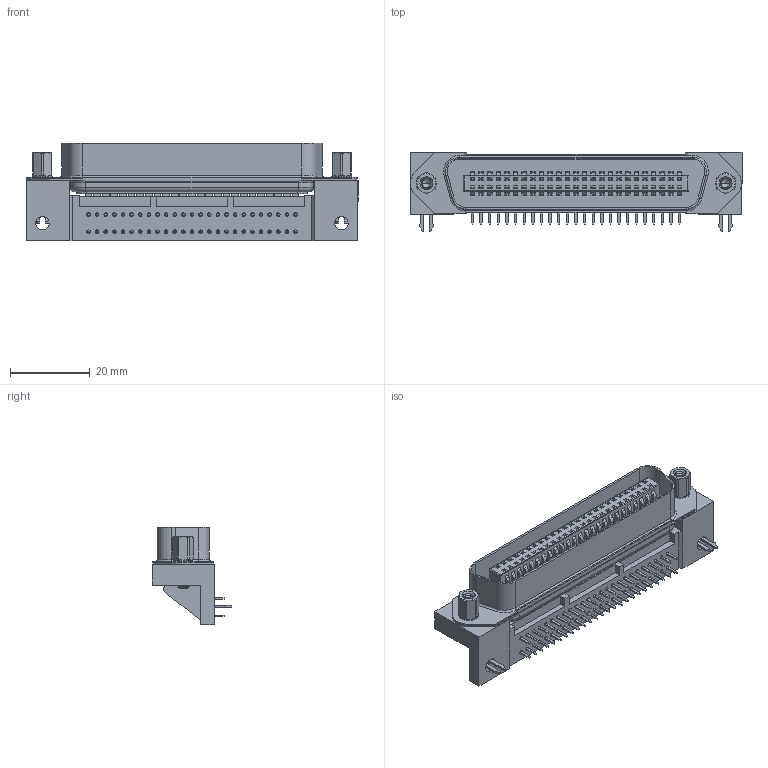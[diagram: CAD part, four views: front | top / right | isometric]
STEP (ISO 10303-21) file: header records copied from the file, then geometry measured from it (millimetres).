
FILE_DESCRIPTION (( 'STEP AP203' ), '1' );
FILE_NAME ('B57-150-661-802.STEP', '2020-06-24T13:16:50', ( '' ), ( '' ), 'SwSTEP 2.0', 'SolidWorks 2020', '' );
FILE_SCHEMA (( 'CONFIG_CONTROL_DESIGN' ));
Length unit declared in the file: millimetre
Products named in the file (9): B57 Front Shell MALE_50 Position UP; B57 Housing Insert MALE_50 Position UP; B57 Board Mount Bracket_BOARDLOCK; B57 RA Housing_50 Position; B57 Rivet_90 THREAD; B57 Hex Standoff; B57-150-661-802; B57 Contacts MALE_50 Position 90 2.54; B57 Back Shell_50 Position
Assembly tree (11 placements, depth 2):
  B57-150-661-802
    B57 Back Shell_50 Position
    B57 RA Housing_50 Position
    B57 Board Mount Bracket_BOARDLOCK  x2
    B57 Rivet_90 THREAD  x2
    B57 Housing Insert MALE_50 Position UP
    B57 Front Shell MALE_50 Position UP
    B57 Contacts MALE_50 Position 90 2.54
    B57 Hex Standoff  x2
Bounding box: 83.1 x 20 x 24.4 mm (x, y, z)
Volume: 9784.3 mm3; surface area: 21182.1 mm2
Topology: 60 solids, 60 shells, 5659 faces, 16391 edges, 10554 vertices
Faces by surface type: plane 3752, cylinder 1509, sphere 204, cone 144, torus 32, bspline 18
Entity records: 184384 total; most frequent: CARTESIAN_POINT 37699, ORIENTED_EDGE 31518, DIRECTION 29101, EDGE_CURVE 15759, VECTOR 12453, LINE 12453, VERTEX_POINT 10276, AXIS2_PLACEMENT_3D 8324
